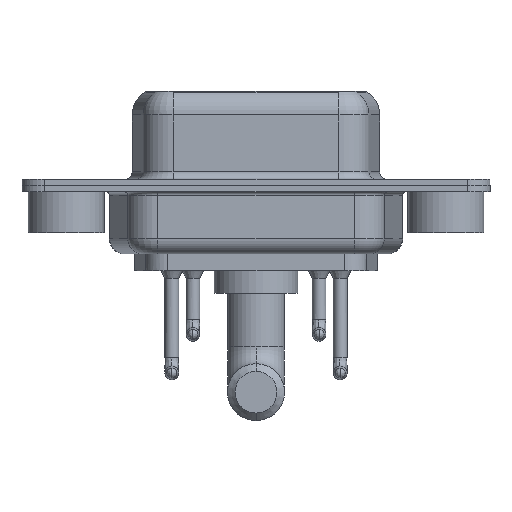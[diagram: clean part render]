
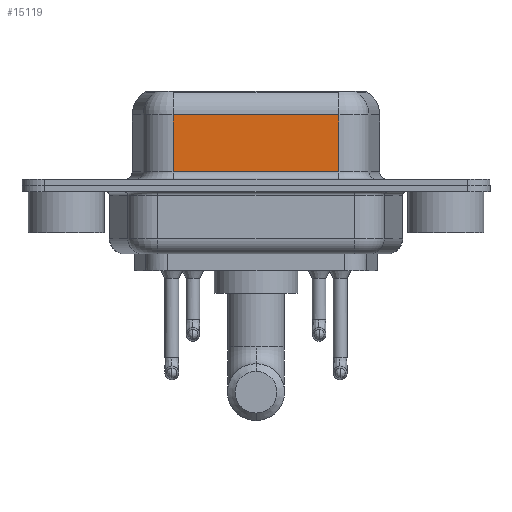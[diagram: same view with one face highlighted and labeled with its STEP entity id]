
A CAD part, front view. The second image highlights one B-rep face of the part: STEP entity #15119.
In plain terms, the highlighted planar face has unit normal (0, -1, 0).
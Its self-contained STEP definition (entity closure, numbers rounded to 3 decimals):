
#863 = CARTESIAN_POINT ( 'NONE',  ( 17.962, -3.95, 0.9 ) ) ;
#869 = DIRECTION ( 'NONE',  ( 0., 1., 0. ) ) ;
#1381 = EDGE_LOOP ( 'NONE', ( #7927, #7982, #1782, #8261 ) ) ;
#1647 = CARTESIAN_POINT ( 'NONE',  ( 17.962, -3.95, 0.9 ) ) ;
#1777 = CARTESIAN_POINT ( 'NONE',  ( 17.962, -3.95, 4.65 ) ) ;
#1782 = ORIENTED_EDGE ( 'NONE', *, *, #9883, .T. ) ;
#2272 = PLANE ( 'NONE',  #12532 ) ;
#3269 = FACE_OUTER_BOUND ( 'NONE', #1381, .T. ) ;
#3449 = CARTESIAN_POINT ( 'NONE',  ( 7.038, -3.95, 6.4 ) ) ;
#3526 = LINE ( 'NONE', #3449, #12872 ) ;
#4825 = DIRECTION ( 'NONE',  ( 1., 0., 0. ) ) ;
#4839 = EDGE_CURVE ( 'NONE', #8115, #6455, #5337, .T. ) ;
#5337 = LINE ( 'NONE', #6663, #10429 ) ;
#5890 = CARTESIAN_POINT ( 'NONE',  ( 17.962, -3.95, 6.4 ) ) ;
#6179 = CARTESIAN_POINT ( 'NONE',  ( 7.038, -3.95, 0.9 ) ) ;
#6455 = VERTEX_POINT ( 'NONE', #1647 ) ;
#6663 = CARTESIAN_POINT ( 'NONE',  ( 17.962, -3.95, 6.4 ) ) ;
#7162 = DIRECTION ( 'NONE',  ( 0., 0., -1. ) ) ;
#7458 = CARTESIAN_POINT ( 'NONE',  ( 7.038, -3.95, 4.65 ) ) ;
#7927 = ORIENTED_EDGE ( 'NONE', *, *, #4839, .F. ) ;
#7982 = ORIENTED_EDGE ( 'NONE', *, *, #12932, .T. ) ;
#8115 = VERTEX_POINT ( 'NONE', #13309 ) ;
#8261 = ORIENTED_EDGE ( 'NONE', *, *, #11710, .T. ) ;
#9883 = EDGE_CURVE ( 'NONE', #13790, #14236, #3526, .T. ) ;
#10429 = VECTOR ( 'NONE', #13952, 1000. ) ;
#10726 = DIRECTION ( 'NONE',  ( -1., 0., 0. ) ) ;
#11054 = LINE ( 'NONE', #863, #12387 ) ;
#11710 = EDGE_CURVE ( 'NONE', #14236, #6455, #11054, .T. ) ;
#12387 = VECTOR ( 'NONE', #4825, 1000. ) ;
#12532 = AXIS2_PLACEMENT_3D ( 'NONE', #5890, #869, #16082 ) ;
#12872 = VECTOR ( 'NONE', #7162, 1000. ) ;
#12932 = EDGE_CURVE ( 'NONE', #8115, #13790, #14341, .T. ) ;
#13309 = CARTESIAN_POINT ( 'NONE',  ( 17.962, -3.95, 4.65 ) ) ;
#13790 = VERTEX_POINT ( 'NONE', #7458 ) ;
#13952 = DIRECTION ( 'NONE',  ( 0., 0., -1. ) ) ;
#14236 = VERTEX_POINT ( 'NONE', #6179 ) ;
#14341 = LINE ( 'NONE', #1777, #14801 ) ;
#14801 = VECTOR ( 'NONE', #10726, 1000. ) ;
#15119 = ADVANCED_FACE ( 'NONE', ( #3269 ), #2272, .F. ) ;
#16082 = DIRECTION ( 'NONE',  ( -1., 0., 0. ) ) ;
